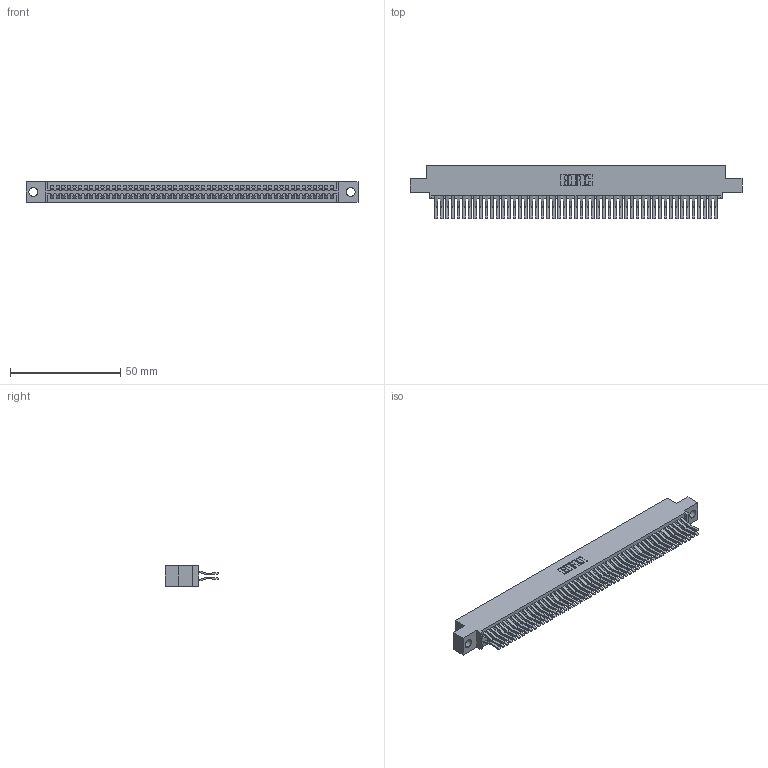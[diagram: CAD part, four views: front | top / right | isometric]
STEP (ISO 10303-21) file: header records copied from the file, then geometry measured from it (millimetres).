
FILE_DESCRIPTION (( 'STEP AP203' ), '1' );
FILE_NAME ('345-102-560-504.STEP', '2021-05-21T13:17:03', ( '' ), ( '' ), 'SwSTEP 2.0', 'SolidWorks 2020', '' );
FILE_SCHEMA (( 'CONFIG_CONTROL_DESIGN' ));
Length unit declared in the file: inch
Products named in the file (3): 345-292-001_560 Tail; 345-102-560-504; 345 Part_0.110 Offset - 0.156 Dia-TI
Assembly tree (103 placements, depth 2):
  345-102-560-504
    345 Part_0.110 Offset - 0.156 Dia-TI
    345-292-001_560 Tail  x102
Bounding box: 150.75 x 24.45 x 9.4 mm (x, y, z)
Volume: 15216.7 mm3; surface area: 24331.1 mm2
Topology: 103 solids, 103 shells, 5448 faces, 16199 edges, 10662 vertices
Faces by surface type: plane 3464, cylinder 1984
Entity records: 39443 total; most frequent: CARTESIAN_POINT 6610, ORIENTED_EDGE 6542, DIRECTION 5819, EDGE_CURVE 3271, LINE 2931, VECTOR 2931, VERTEX_POINT 2178, AXIS2_PLACEMENT_3D 1444
